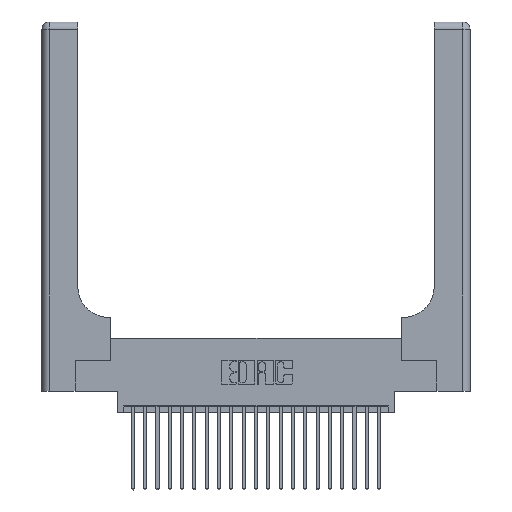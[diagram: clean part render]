
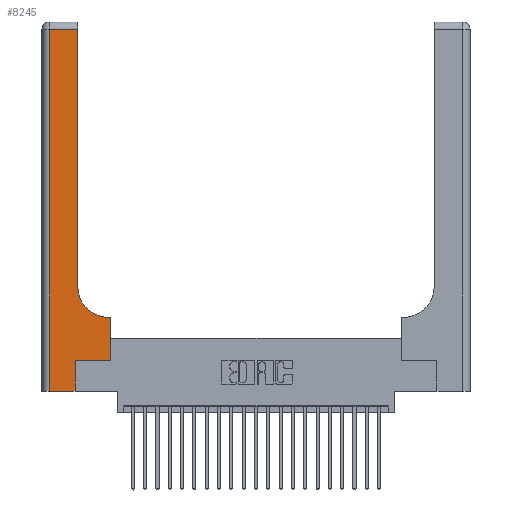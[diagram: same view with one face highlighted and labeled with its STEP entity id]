
A CAD part, top view. The second image highlights one B-rep face of the part: STEP entity #8245.
In plain terms, the highlighted planar face has unit normal (0, 0, 1).
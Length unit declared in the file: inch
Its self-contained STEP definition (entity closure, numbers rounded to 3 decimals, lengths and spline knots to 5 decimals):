
#394 = CARTESIAN_POINT ( 'NONE',  ( 0.06, 0., 0.37 ) ) ;
#1008 = EDGE_LOOP ( 'NONE', ( #8898, #3306, #24069, #12583, #18202, #12672, #4506, #16155, #24617 ) ) ;
#1090 = VECTOR ( 'NONE', #5242, 39.37008 ) ;
#2344 = LINE ( 'NONE', #5768, #15153 ) ;
#2381 = CARTESIAN_POINT ( 'NONE',  ( 0.5585, 0.25, 0.37 ) ) ;
#2760 = CARTESIAN_POINT ( 'NONE',  ( 0., 2.94, 0.37 ) ) ;
#2774 = CARTESIAN_POINT ( 'NONE',  ( 0., 0., 0.37 ) ) ;
#2867 = EDGE_CURVE ( 'NONE', #5373, #13496, #17671, .T. ) ;
#3306 = ORIENTED_EDGE ( 'NONE', *, *, #2867, .T. ) ;
#3616 = PLANE ( 'NONE',  #12087 ) ;
#3771 = CARTESIAN_POINT ( 'NONE',  ( 0.5415, 0.85, 0.37 ) ) ;
#3977 = DIRECTION ( 'NONE',  ( 1., 0., 0. ) ) ;
#4219 = EDGE_CURVE ( 'NONE', #9874, #12159, #19354, .T. ) ;
#4477 = CARTESIAN_POINT ( 'NONE',  ( 0.5585, 0.6, 0.37 ) ) ;
#4503 = CARTESIAN_POINT ( 'NONE',  ( 0.269, 0.25, 0.37 ) ) ;
#4506 = ORIENTED_EDGE ( 'NONE', *, *, #19175, .T. ) ;
#4867 = VECTOR ( 'NONE', #6144, 39.37008 ) ;
#5242 = DIRECTION ( 'NONE',  ( 0., 1., 0. ) ) ;
#5373 = VERTEX_POINT ( 'NONE', #7934 ) ;
#5768 = CARTESIAN_POINT ( 'NONE',  ( 0.269, 0., 0.37 ) ) ;
#6017 = EDGE_CURVE ( 'NONE', #12841, #10099, #23016, .T. ) ;
#6144 = DIRECTION ( 'NONE',  ( 0., 1., 0. ) ) ;
#6580 = FACE_OUTER_BOUND ( 'NONE', #1008, .T. ) ;
#7835 = VECTOR ( 'NONE', #3977, 39.37008 ) ;
#7934 = CARTESIAN_POINT ( 'NONE',  ( 0.2915, 2.94, 0.37 ) ) ;
#7936 = DIRECTION ( 'NONE',  ( 0., 0., -1. ) ) ;
#7959 = CARTESIAN_POINT ( 'NONE',  ( 0.269, 0., 0.37 ) ) ;
#8178 = DIRECTION ( 'NONE',  ( -1., 0., 0. ) ) ;
#8245 = ADVANCED_FACE ( 'NONE', ( #6580 ), #3616, .F. ) ;
#8898 = ORIENTED_EDGE ( 'NONE', *, *, #12102, .T. ) ;
#9182 = VECTOR ( 'NONE', #23986, 39.37008 ) ;
#9776 = LINE ( 'NONE', #12925, #9182 ) ;
#9874 = VERTEX_POINT ( 'NONE', #394 ) ;
#10088 = CARTESIAN_POINT ( 'NONE',  ( 0.2915, 0.85, 0.37 ) ) ;
#10099 = VERTEX_POINT ( 'NONE', #2381 ) ;
#10341 = AXIS2_PLACEMENT_3D ( 'NONE', #3771, #19216, #17171 ) ;
#11030 = CARTESIAN_POINT ( 'NONE',  ( 0.5415, 0.6, 0.37 ) ) ;
#11531 = CIRCLE ( 'NONE', #10341, 0.25 ) ;
#11620 = VERTEX_POINT ( 'NONE', #4477 ) ;
#12087 = AXIS2_PLACEMENT_3D ( 'NONE', #20645, #7936, #15417 ) ;
#12102 = EDGE_CURVE ( 'NONE', #16667, #5373, #19414, .T. ) ;
#12159 = VERTEX_POINT ( 'NONE', #7959 ) ;
#12583 = ORIENTED_EDGE ( 'NONE', *, *, #4219, .T. ) ;
#12672 = ORIENTED_EDGE ( 'NONE', *, *, #6017, .T. ) ;
#12841 = VERTEX_POINT ( 'NONE', #4503 ) ;
#12925 = CARTESIAN_POINT ( 'NONE',  ( 0.2915, 0.6, 0.37 ) ) ;
#13000 = LINE ( 'NONE', #23969, #1090 ) ;
#13191 = VECTOR ( 'NONE', #23268, 39.37008 ) ;
#13265 = EDGE_CURVE ( 'NONE', #13496, #9874, #23916, .T. ) ;
#13496 = VERTEX_POINT ( 'NONE', #16899 ) ;
#13923 = DIRECTION ( 'NONE',  ( 1., 0., 0. ) ) ;
#15021 = VECTOR ( 'NONE', #8178, 39.37008 ) ;
#15153 = VECTOR ( 'NONE', #17322, 39.37008 ) ;
#15417 = DIRECTION ( 'NONE',  ( -1., 0., 0. ) ) ;
#15915 = EDGE_CURVE ( 'NONE', #12159, #12841, #2344, .T. ) ;
#16155 = ORIENTED_EDGE ( 'NONE', *, *, #16340, .T. ) ;
#16340 = EDGE_CURVE ( 'NONE', #11620, #23625, #9776, .T. ) ;
#16667 = VERTEX_POINT ( 'NONE', #10088 ) ;
#16899 = CARTESIAN_POINT ( 'NONE',  ( 0.06, 2.94, 0.37 ) ) ;
#17171 = DIRECTION ( 'NONE',  ( 1., 0., 0. ) ) ;
#17322 = DIRECTION ( 'NONE',  ( 0., 1., 0. ) ) ;
#17595 = VECTOR ( 'NONE', #13923, 39.37008 ) ;
#17671 = LINE ( 'NONE', #2760, #15021 ) ;
#18202 = ORIENTED_EDGE ( 'NONE', *, *, #15915, .T. ) ;
#19175 = EDGE_CURVE ( 'NONE', #10099, #11620, #13000, .T. ) ;
#19216 = DIRECTION ( 'NONE',  ( 0., 0., -1. ) ) ;
#19354 = LINE ( 'NONE', #2774, #17595 ) ;
#19414 = LINE ( 'NONE', #21075, #4867 ) ;
#20645 = CARTESIAN_POINT ( 'NONE',  ( 0., 3., 0.37 ) ) ;
#21075 = CARTESIAN_POINT ( 'NONE',  ( 0.2915, 3., 0.37 ) ) ;
#21151 = EDGE_CURVE ( 'NONE', #23625, #16667, #11531, .T. ) ;
#21178 = CARTESIAN_POINT ( 'NONE',  ( 0.269, 0.25, 0.37 ) ) ;
#21235 = CARTESIAN_POINT ( 'NONE',  ( 0.06, 3., 0.37 ) ) ;
#23016 = LINE ( 'NONE', #21178, #7835 ) ;
#23268 = DIRECTION ( 'NONE',  ( 0., -1., 0. ) ) ;
#23625 = VERTEX_POINT ( 'NONE', #11030 ) ;
#23916 = LINE ( 'NONE', #21235, #13191 ) ;
#23969 = CARTESIAN_POINT ( 'NONE',  ( 0.5585, 0.25, 0.37 ) ) ;
#23986 = DIRECTION ( 'NONE',  ( -1., 0., 0. ) ) ;
#24069 = ORIENTED_EDGE ( 'NONE', *, *, #13265, .T. ) ;
#24617 = ORIENTED_EDGE ( 'NONE', *, *, #21151, .T. ) ;
